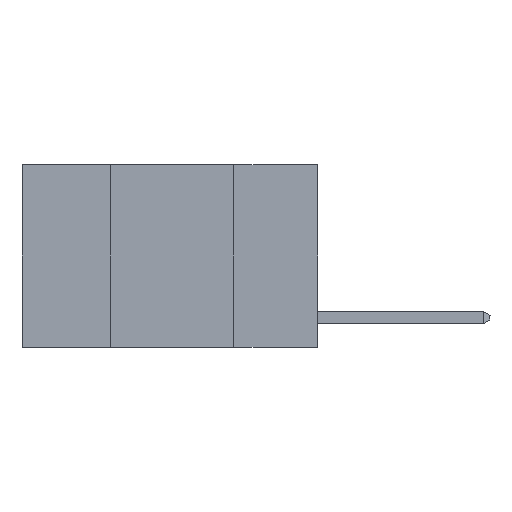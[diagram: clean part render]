
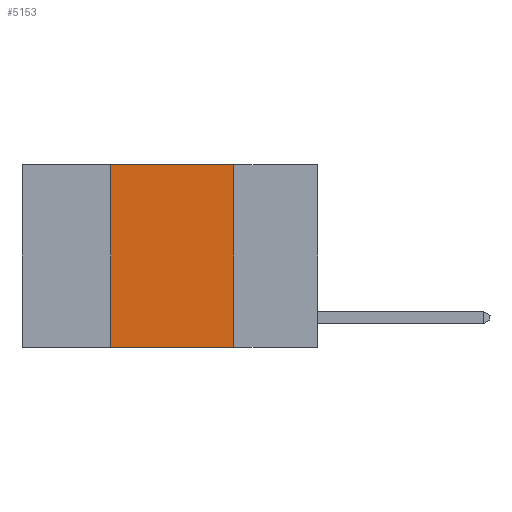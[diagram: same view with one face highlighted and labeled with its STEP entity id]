
A CAD part, left-side view. The second image highlights one B-rep face of the part: STEP entity #5153.
In plain terms, the highlighted planar face has unit normal (-1, 0, 0).
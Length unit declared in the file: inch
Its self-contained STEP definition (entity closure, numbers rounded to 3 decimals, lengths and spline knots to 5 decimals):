
#132 = CARTESIAN_POINT ( 'NONE',  ( 0., 0.17, 0. ) ) ;
#139 = ORIENTED_EDGE ( 'NONE', *, *, #353, .F. ) ;
#353 = EDGE_CURVE ( 'NONE', #7822, #2926, #10407, .T. ) ;
#635 = VERTEX_POINT ( 'NONE', #1475 ) ;
#922 = VERTEX_POINT ( 'NONE', #1453 ) ;
#1058 = ORIENTED_EDGE ( 'NONE', *, *, #8876, .F. ) ;
#1320 = EDGE_LOOP ( 'NONE', ( #4835, #1058, #139, #9534 ) ) ;
#1405 = VECTOR ( 'NONE', #1738, 39.37008 ) ;
#1453 = CARTESIAN_POINT ( 'NONE',  ( 0., 0.17, 0. ) ) ;
#1475 = CARTESIAN_POINT ( 'NONE',  ( 0., 0.17, -0.37 ) ) ;
#1738 = DIRECTION ( 'NONE',  ( 0., 0., 1. ) ) ;
#1968 = CARTESIAN_POINT ( 'NONE',  ( 0., 0.6, -0.37 ) ) ;
#2441 = LINE ( 'NONE', #8181, #9609 ) ;
#2502 = PLANE ( 'NONE',  #5395 ) ;
#2851 = LINE ( 'NONE', #1968, #8987 ) ;
#2926 = VERTEX_POINT ( 'NONE', #7435 ) ;
#3156 = CARTESIAN_POINT ( 'NONE',  ( 0., 0.42, 0. ) ) ;
#3214 = DIRECTION ( 'NONE',  ( 0., 0., -1. ) ) ;
#3809 = EDGE_CURVE ( 'NONE', #7822, #635, #2851, .T. ) ;
#4835 = ORIENTED_EDGE ( 'NONE', *, *, #7771, .F. ) ;
#4979 = DIRECTION ( 'NONE',  ( 1., 0., 0. ) ) ;
#5153 = ADVANCED_FACE ( 'NONE', ( #6530 ), #2502, .F. ) ;
#5395 = AXIS2_PLACEMENT_3D ( 'NONE', #7208, #4979, #3214 ) ;
#5789 = VECTOR ( 'NONE', #8218, 39.37008 ) ;
#6072 = DIRECTION ( 'NONE',  ( 0., -1., 0. ) ) ;
#6530 = FACE_OUTER_BOUND ( 'NONE', #1320, .T. ) ;
#7208 = CARTESIAN_POINT ( 'NONE',  ( 0., 0.6, 0. ) ) ;
#7435 = CARTESIAN_POINT ( 'NONE',  ( 0., 0.42, 0. ) ) ;
#7771 = EDGE_CURVE ( 'NONE', #922, #635, #8171, .T. ) ;
#7822 = VERTEX_POINT ( 'NONE', #7877 ) ;
#7877 = CARTESIAN_POINT ( 'NONE',  ( 0., 0.42, -0.37 ) ) ;
#8171 = LINE ( 'NONE', #132, #5789 ) ;
#8181 = CARTESIAN_POINT ( 'NONE',  ( 0., 0.6, 0. ) ) ;
#8218 = DIRECTION ( 'NONE',  ( 0., 0., -1. ) ) ;
#8876 = EDGE_CURVE ( 'NONE', #2926, #922, #2441, .T. ) ;
#8915 = DIRECTION ( 'NONE',  ( 0., -1., 0. ) ) ;
#8987 = VECTOR ( 'NONE', #6072, 39.37008 ) ;
#9534 = ORIENTED_EDGE ( 'NONE', *, *, #3809, .T. ) ;
#9609 = VECTOR ( 'NONE', #8915, 39.37008 ) ;
#10407 = LINE ( 'NONE', #3156, #1405 ) ;
